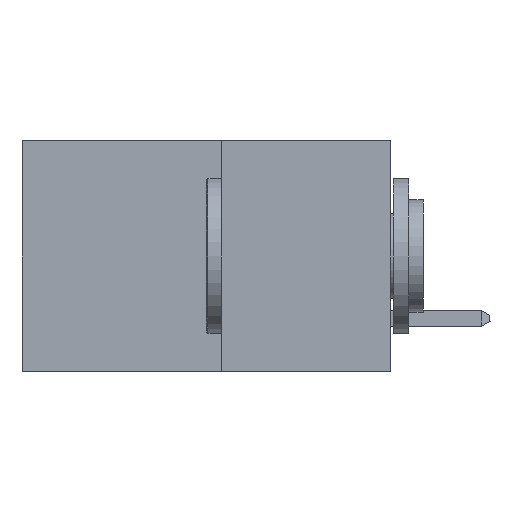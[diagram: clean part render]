
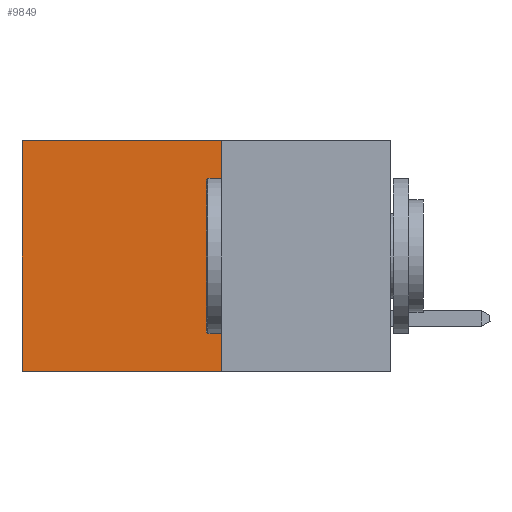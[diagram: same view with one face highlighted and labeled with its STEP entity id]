
A CAD part, left-side view. The second image highlights one B-rep face of the part: STEP entity #9849.
In plain terms, the highlighted planar face has unit normal (-1, 0, 0).
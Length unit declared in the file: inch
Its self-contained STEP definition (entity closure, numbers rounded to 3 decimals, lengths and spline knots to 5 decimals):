
#32 = DIRECTION ( 'NONE',  ( 0., 1., 0. ) ) ;
#415 = PLANE ( 'NONE',  #10367 ) ;
#449 = ORIENTED_EDGE ( 'NONE', *, *, #13444, .T. ) ;
#600 = DIRECTION ( 'NONE',  ( 0., 1., 0. ) ) ;
#2059 = VERTEX_POINT ( 'NONE', #12505 ) ;
#2192 = CARTESIAN_POINT ( 'NONE',  ( 0.277, 0.27, -0.37 ) ) ;
#2861 = VERTEX_POINT ( 'NONE', #3759 ) ;
#3183 = EDGE_CURVE ( 'NONE', #2059, #6152, #11760, .T. ) ;
#3759 = CARTESIAN_POINT ( 'NONE',  ( 0.277, 0.59, 0. ) ) ;
#3810 = VECTOR ( 'NONE', #32, 39.37008 ) ;
#4312 = EDGE_LOOP ( 'NONE', ( #7573, #7852, #8198, #449 ) ) ;
#4415 = CARTESIAN_POINT ( 'NONE',  ( 0.277, 0.27, -0.37 ) ) ;
#5277 = CARTESIAN_POINT ( 'NONE',  ( 0.277, 0.27, 0. ) ) ;
#5810 = DIRECTION ( 'NONE',  ( 0., 0., -1. ) ) ;
#6034 = EDGE_CURVE ( 'NONE', #2861, #6152, #7208, .T. ) ;
#6152 = VERTEX_POINT ( 'NONE', #8237 ) ;
#7208 = LINE ( 'NONE', #8822, #13683 ) ;
#7431 = VECTOR ( 'NONE', #11618, 39.37008 ) ;
#7455 = CARTESIAN_POINT ( 'NONE',  ( 0.277, 0.27, 0. ) ) ;
#7573 = ORIENTED_EDGE ( 'NONE', *, *, #6034, .T. ) ;
#7852 = ORIENTED_EDGE ( 'NONE', *, *, #3183, .F. ) ;
#7859 = LINE ( 'NONE', #2192, #7431 ) ;
#8198 = ORIENTED_EDGE ( 'NONE', *, *, #9416, .F. ) ;
#8237 = CARTESIAN_POINT ( 'NONE',  ( 0.277, 0.59, -0.37 ) ) ;
#8735 = DIRECTION ( 'NONE',  ( 0., 0., -1. ) ) ;
#8822 = CARTESIAN_POINT ( 'NONE',  ( 0.277, 0.59, -0.37 ) ) ;
#9416 = EDGE_CURVE ( 'NONE', #16692, #2059, #7859, .T. ) ;
#9849 = ADVANCED_FACE ( 'NONE', ( #10477 ), #415, .F. ) ;
#10367 = AXIS2_PLACEMENT_3D ( 'NONE', #4415, #13651, #5810 ) ;
#10477 = FACE_OUTER_BOUND ( 'NONE', #4312, .T. ) ;
#10632 = LINE ( 'NONE', #7455, #13616 ) ;
#11618 = DIRECTION ( 'NONE',  ( 0., 0., -1. ) ) ;
#11760 = LINE ( 'NONE', #11810, #3810 ) ;
#11810 = CARTESIAN_POINT ( 'NONE',  ( 0.277, 0.27, -0.37 ) ) ;
#12505 = CARTESIAN_POINT ( 'NONE',  ( 0.277, 0.27, -0.37 ) ) ;
#13444 = EDGE_CURVE ( 'NONE', #16692, #2861, #10632, .T. ) ;
#13616 = VECTOR ( 'NONE', #600, 39.37008 ) ;
#13651 = DIRECTION ( 'NONE',  ( 1., 0., 0. ) ) ;
#13683 = VECTOR ( 'NONE', #8735, 39.37008 ) ;
#16692 = VERTEX_POINT ( 'NONE', #5277 ) ;
